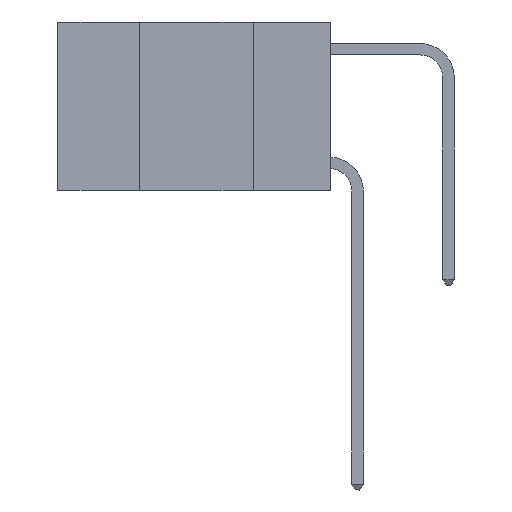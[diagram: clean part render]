
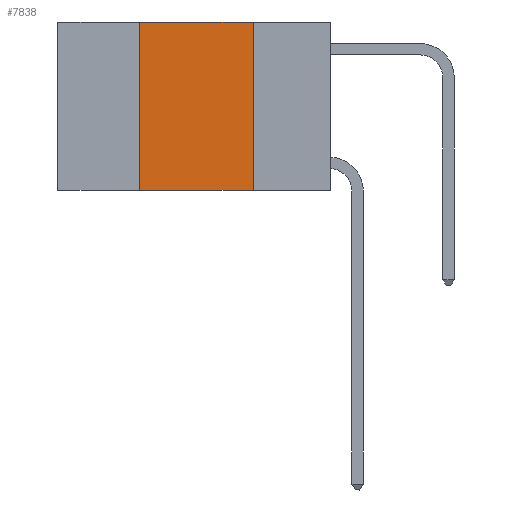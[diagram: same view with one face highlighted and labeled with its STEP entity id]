
A CAD part, left-side view. The second image highlights one B-rep face of the part: STEP entity #7838.
In plain terms, the highlighted planar face has unit normal (-1, 0, 0).
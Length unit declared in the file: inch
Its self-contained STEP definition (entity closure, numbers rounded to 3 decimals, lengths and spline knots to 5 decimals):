
#87 = VECTOR ( 'NONE', #8087, 39.37008 ) ;
#141 = LINE ( 'NONE', #9253, #3207 ) ;
#258 = ORIENTED_EDGE ( 'NONE', *, *, #10735, .F. ) ;
#277 = FACE_OUTER_BOUND ( 'NONE', #6267, .T. ) ;
#531 = VERTEX_POINT ( 'NONE', #6157 ) ;
#1306 = VERTEX_POINT ( 'NONE', #11034 ) ;
#1347 = EDGE_CURVE ( 'NONE', #8058, #2772, #141, .T. ) ;
#2241 = DIRECTION ( 'NONE',  ( 1., 0., 0. ) ) ;
#2399 = CARTESIAN_POINT ( 'NONE',  ( 0., 0.6, 0. ) ) ;
#2444 = DIRECTION ( 'NONE',  ( 0., -1., 0. ) ) ;
#2718 = ORIENTED_EDGE ( 'NONE', *, *, #4932, .F. ) ;
#2772 = VERTEX_POINT ( 'NONE', #7273 ) ;
#3154 = DIRECTION ( 'NONE',  ( 0., 0., -1. ) ) ;
#3207 = VECTOR ( 'NONE', #4017, 39.37008 ) ;
#4017 = DIRECTION ( 'NONE',  ( 0., -1., 0. ) ) ;
#4107 = AXIS2_PLACEMENT_3D ( 'NONE', #8282, #2241, #10887 ) ;
#4113 = LINE ( 'NONE', #7269, #87 ) ;
#4117 = CARTESIAN_POINT ( 'NONE',  ( 0., 0.17, 0. ) ) ;
#4932 = EDGE_CURVE ( 'NONE', #1306, #531, #9720, .T. ) ;
#5264 = VECTOR ( 'NONE', #3154, 39.37008 ) ;
#5444 = ORIENTED_EDGE ( 'NONE', *, *, #1347, .T. ) ;
#6157 = CARTESIAN_POINT ( 'NONE',  ( 0., 0.17, 0. ) ) ;
#6267 = EDGE_LOOP ( 'NONE', ( #258, #2718, #9778, #5444 ) ) ;
#7269 = CARTESIAN_POINT ( 'NONE',  ( 0., 0.42, 0. ) ) ;
#7273 = CARTESIAN_POINT ( 'NONE',  ( 0., 0.17, -0.37 ) ) ;
#7838 = ADVANCED_FACE ( 'NONE', ( #277 ), #9307, .F. ) ;
#8058 = VERTEX_POINT ( 'NONE', #8237 ) ;
#8087 = DIRECTION ( 'NONE',  ( 0., 0., 1. ) ) ;
#8237 = CARTESIAN_POINT ( 'NONE',  ( 0., 0.42, -0.37 ) ) ;
#8282 = CARTESIAN_POINT ( 'NONE',  ( 0., 0.6, 0. ) ) ;
#8954 = LINE ( 'NONE', #4117, #5264 ) ;
#9055 = EDGE_CURVE ( 'NONE', #8058, #1306, #4113, .T. ) ;
#9253 = CARTESIAN_POINT ( 'NONE',  ( 0., 0.6, -0.37 ) ) ;
#9307 = PLANE ( 'NONE',  #4107 ) ;
#9720 = LINE ( 'NONE', #2399, #10129 ) ;
#9778 = ORIENTED_EDGE ( 'NONE', *, *, #9055, .F. ) ;
#10129 = VECTOR ( 'NONE', #2444, 39.37008 ) ;
#10735 = EDGE_CURVE ( 'NONE', #531, #2772, #8954, .T. ) ;
#10887 = DIRECTION ( 'NONE',  ( 0., 0., -1. ) ) ;
#11034 = CARTESIAN_POINT ( 'NONE',  ( 0., 0.42, 0. ) ) ;
